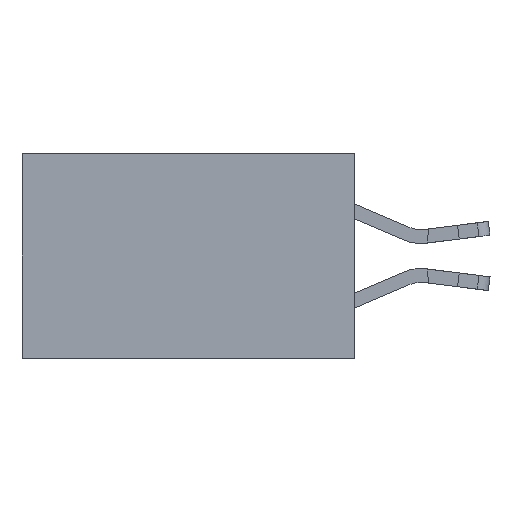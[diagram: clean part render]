
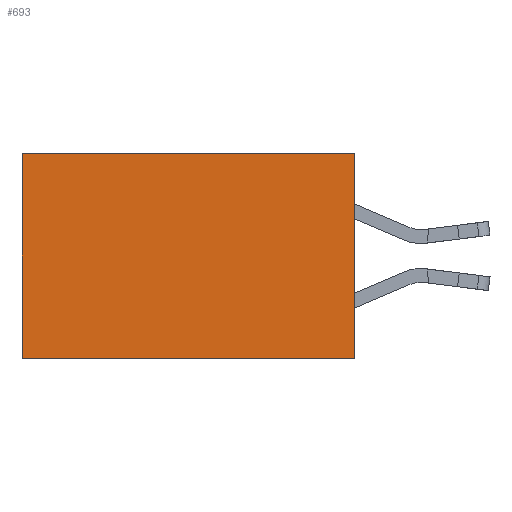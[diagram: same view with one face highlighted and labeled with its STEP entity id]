
A CAD part, left-side view. The second image highlights one B-rep face of the part: STEP entity #693.
In plain terms, the highlighted planar face has unit normal (-1, 0, 0).
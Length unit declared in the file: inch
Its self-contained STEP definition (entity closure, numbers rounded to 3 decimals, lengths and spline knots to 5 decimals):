
#589 = VECTOR ( 'NONE', #5667, 39.37008 ) ;
#693 = ADVANCED_FACE ( 'NONE', ( #23249 ), #11884, .F. ) ;
#1191 = ORIENTED_EDGE ( 'NONE', *, *, #6122, .F. ) ;
#1747 = LINE ( 'NONE', #11615, #20085 ) ;
#1754 = AXIS2_PLACEMENT_3D ( 'NONE', #25758, #13651, #26024 ) ;
#2177 = CARTESIAN_POINT ( 'NONE',  ( 0.298, 0., 0. ) ) ;
#4318 = LINE ( 'NONE', #11896, #19820 ) ;
#5667 = DIRECTION ( 'NONE',  ( 0., 1., 0. ) ) ;
#6122 = EDGE_CURVE ( 'NONE', #8882, #14389, #19898, .T. ) ;
#8882 = VERTEX_POINT ( 'NONE', #22882 ) ;
#10244 = CARTESIAN_POINT ( 'NONE',  ( 0.298, 0.6, -0.37 ) ) ;
#11615 = CARTESIAN_POINT ( 'NONE',  ( 0.298, 0., 0. ) ) ;
#11884 = PLANE ( 'NONE',  #1754 ) ;
#11896 = CARTESIAN_POINT ( 'NONE',  ( 0.298, 0.6, 0. ) ) ;
#12184 = CARTESIAN_POINT ( 'NONE',  ( 0.298, 0., 0. ) ) ;
#13494 = EDGE_LOOP ( 'NONE', ( #24422, #1191, #21411, #24511 ) ) ;
#13501 = EDGE_CURVE ( 'NONE', #21470, #14389, #4318, .T. ) ;
#13651 = DIRECTION ( 'NONE',  ( 1., 0., 0. ) ) ;
#13653 = DIRECTION ( 'NONE',  ( 0., 1., 0. ) ) ;
#14389 = VERTEX_POINT ( 'NONE', #10244 ) ;
#16180 = CARTESIAN_POINT ( 'NONE',  ( 0.298, 0., -0.37 ) ) ;
#16298 = DIRECTION ( 'NONE',  ( 0., 0., -1. ) ) ;
#18893 = EDGE_CURVE ( 'NONE', #22543, #21470, #1747, .T. ) ;
#19367 = VECTOR ( 'NONE', #16298, 39.37008 ) ;
#19820 = VECTOR ( 'NONE', #21618, 39.37008 ) ;
#19898 = LINE ( 'NONE', #16180, #589 ) ;
#20085 = VECTOR ( 'NONE', #13653, 39.37008 ) ;
#21411 = ORIENTED_EDGE ( 'NONE', *, *, #24323, .F. ) ;
#21470 = VERTEX_POINT ( 'NONE', #22734 ) ;
#21618 = DIRECTION ( 'NONE',  ( 0., 0., -1. ) ) ;
#22543 = VERTEX_POINT ( 'NONE', #12184 ) ;
#22734 = CARTESIAN_POINT ( 'NONE',  ( 0.298, 0.6, 0. ) ) ;
#22882 = CARTESIAN_POINT ( 'NONE',  ( 0.298, 0., -0.37 ) ) ;
#23249 = FACE_OUTER_BOUND ( 'NONE', #13494, .T. ) ;
#24323 = EDGE_CURVE ( 'NONE', #22543, #8882, #24732, .T. ) ;
#24422 = ORIENTED_EDGE ( 'NONE', *, *, #13501, .T. ) ;
#24511 = ORIENTED_EDGE ( 'NONE', *, *, #18893, .T. ) ;
#24732 = LINE ( 'NONE', #2177, #19367 ) ;
#25758 = CARTESIAN_POINT ( 'NONE',  ( 0.298, 0., 0. ) ) ;
#26024 = DIRECTION ( 'NONE',  ( 0., 0., -1. ) ) ;
